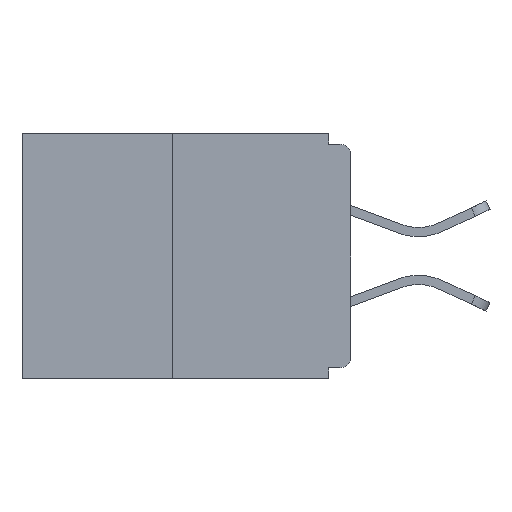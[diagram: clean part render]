
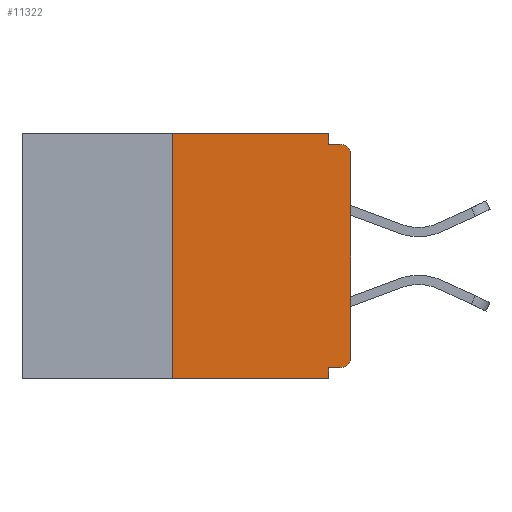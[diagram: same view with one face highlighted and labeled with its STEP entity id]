
A CAD part, left-side view. The second image highlights one B-rep face of the part: STEP entity #11322.
In plain terms, the highlighted planar face has unit normal (-1, 0, 0).
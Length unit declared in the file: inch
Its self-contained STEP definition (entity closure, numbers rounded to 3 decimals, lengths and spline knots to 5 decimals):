
#117 = DIRECTION ( 'NONE',  ( -1., 0., 0. ) ) ;
#404 = AXIS2_PLACEMENT_3D ( 'NONE', #14959, #117, #7440 ) ;
#451 = ORIENTED_EDGE ( 'NONE', *, *, #8232, .F. ) ;
#1149 = ORIENTED_EDGE ( 'NONE', *, *, #3819, .F. ) ;
#1339 = ORIENTED_EDGE ( 'NONE', *, *, #10463, .T. ) ;
#1766 = VERTEX_POINT ( 'NONE', #9526 ) ;
#1997 = VERTEX_POINT ( 'NONE', #14648 ) ;
#2332 = EDGE_CURVE ( 'NONE', #9503, #16705, #18944, .T. ) ;
#2663 = EDGE_LOOP ( 'NONE', ( #12184, #16238, #3317, #6544, #1149, #1339, #11304, #2722, #451, #3646 ) ) ;
#2677 = CARTESIAN_POINT ( 'NONE',  ( 0., 0.031, -0.328 ) ) ;
#2722 = ORIENTED_EDGE ( 'NONE', *, *, #17305, .T. ) ;
#2794 = CARTESIAN_POINT ( 'NONE',  ( 0., 0.46, -0.343 ) ) ;
#2967 = VERTEX_POINT ( 'NONE', #2677 ) ;
#3242 = VECTOR ( 'NONE', #5401, 39.37008 ) ;
#3317 = ORIENTED_EDGE ( 'NONE', *, *, #12271, .T. ) ;
#3443 = AXIS2_PLACEMENT_3D ( 'NONE', #6434, #9152, #13773 ) ;
#3646 = ORIENTED_EDGE ( 'NONE', *, *, #4870, .F. ) ;
#3714 = VERTEX_POINT ( 'NONE', #4981 ) ;
#3819 = EDGE_CURVE ( 'NONE', #1997, #2967, #16597, .T. ) ;
#4604 = CARTESIAN_POINT ( 'NONE',  ( 0., 0.031, -0.015 ) ) ;
#4810 = DIRECTION ( 'NONE',  ( 0., -1., 0. ) ) ;
#4870 = EDGE_CURVE ( 'NONE', #1766, #17278, #15366, .T. ) ;
#4981 = CARTESIAN_POINT ( 'NONE',  ( 0., 0., -0.313 ) ) ;
#5036 = CARTESIAN_POINT ( 'NONE',  ( 0., 0.031, -0.343 ) ) ;
#5191 = DIRECTION ( 'NONE',  ( 0., 0., 1. ) ) ;
#5307 = VERTEX_POINT ( 'NONE', #18093 ) ;
#5401 = DIRECTION ( 'NONE',  ( 0., -1., 0. ) ) ;
#5493 = VECTOR ( 'NONE', #6593, 39.37008 ) ;
#5878 = CARTESIAN_POINT ( 'NONE',  ( 0., 0.25, 0. ) ) ;
#6434 = CARTESIAN_POINT ( 'NONE',  ( 0., 0.015, -0.03 ) ) ;
#6523 = CARTESIAN_POINT ( 'NONE',  ( 0., 0.031, 0. ) ) ;
#6544 = ORIENTED_EDGE ( 'NONE', *, *, #14697, .F. ) ;
#6593 = DIRECTION ( 'NONE',  ( 0., 0., -1. ) ) ;
#7440 = DIRECTION ( 'NONE',  ( 0., 0., -1. ) ) ;
#7446 = AXIS2_PLACEMENT_3D ( 'NONE', #12922, #14546, #10168 ) ;
#7646 = LINE ( 'NONE', #14327, #3242 ) ;
#7720 = CARTESIAN_POINT ( 'NONE',  ( 0., 0., -0.015 ) ) ;
#8051 = CIRCLE ( 'NONE', #3443, 0.015 ) ;
#8120 = VECTOR ( 'NONE', #15920, 39.37008 ) ;
#8232 = EDGE_CURVE ( 'NONE', #17278, #5307, #15681, .T. ) ;
#8973 = VECTOR ( 'NONE', #17802, 39.37008 ) ;
#9098 = EDGE_CURVE ( 'NONE', #16705, #1766, #7646, .T. ) ;
#9130 = LINE ( 'NONE', #18225, #18767 ) ;
#9152 = DIRECTION ( 'NONE',  ( -1., 0., 0. ) ) ;
#9433 = LINE ( 'NONE', #14816, #8973 ) ;
#9503 = VERTEX_POINT ( 'NONE', #17490 ) ;
#9526 = CARTESIAN_POINT ( 'NONE',  ( 0., 0.031, 0. ) ) ;
#10168 = DIRECTION ( 'NONE',  ( 0., 0., -1. ) ) ;
#10463 = EDGE_CURVE ( 'NONE', #1997, #3714, #18842, .T. ) ;
#10589 = VERTEX_POINT ( 'NONE', #5036 ) ;
#10707 = FACE_OUTER_BOUND ( 'NONE', #2663, .T. ) ;
#11304 = ORIENTED_EDGE ( 'NONE', *, *, #18548, .T. ) ;
#11322 = ADVANCED_FACE ( 'NONE', ( #10707 ), #17408, .F. ) ;
#11354 = VECTOR ( 'NONE', #11773, 39.37008 ) ;
#11773 = DIRECTION ( 'NONE',  ( 0., 0., 1. ) ) ;
#12184 = ORIENTED_EDGE ( 'NONE', *, *, #9098, .F. ) ;
#12271 = EDGE_CURVE ( 'NONE', #9503, #10589, #17094, .T. ) ;
#12639 = CARTESIAN_POINT ( 'NONE',  ( 0., 0., -0.03 ) ) ;
#12886 = CARTESIAN_POINT ( 'NONE',  ( 0., 0.25, 0. ) ) ;
#12922 = CARTESIAN_POINT ( 'NONE',  ( 0., 0.46, 0. ) ) ;
#13773 = DIRECTION ( 'NONE',  ( 0., 0., -1. ) ) ;
#14327 = CARTESIAN_POINT ( 'NONE',  ( 0., 0.46, 0. ) ) ;
#14546 = DIRECTION ( 'NONE',  ( 1., 0., 0. ) ) ;
#14590 = CARTESIAN_POINT ( 'NONE',  ( 0., 0., -0.328 ) ) ;
#14591 = VECTOR ( 'NONE', #15901, 39.37008 ) ;
#14648 = CARTESIAN_POINT ( 'NONE',  ( 0., 0.015, -0.328 ) ) ;
#14697 = EDGE_CURVE ( 'NONE', #2967, #10589, #9433, .T. ) ;
#14816 = CARTESIAN_POINT ( 'NONE',  ( 0., 0.031, -0.343 ) ) ;
#14959 = CARTESIAN_POINT ( 'NONE',  ( 0., 0.015, -0.313 ) ) ;
#15366 = LINE ( 'NONE', #6523, #5493 ) ;
#15681 = LINE ( 'NONE', #7720, #16832 ) ;
#15901 = DIRECTION ( 'NONE',  ( 0., -1., 0. ) ) ;
#15920 = DIRECTION ( 'NONE',  ( 0., 1., 0. ) ) ;
#16238 = ORIENTED_EDGE ( 'NONE', *, *, #2332, .F. ) ;
#16597 = LINE ( 'NONE', #14590, #8120 ) ;
#16705 = VERTEX_POINT ( 'NONE', #12886 ) ;
#16832 = VECTOR ( 'NONE', #4810, 39.37008 ) ;
#17094 = LINE ( 'NONE', #2794, #14591 ) ;
#17278 = VERTEX_POINT ( 'NONE', #4604 ) ;
#17305 = EDGE_CURVE ( 'NONE', #18595, #5307, #8051, .T. ) ;
#17408 = PLANE ( 'NONE',  #7446 ) ;
#17490 = CARTESIAN_POINT ( 'NONE',  ( 0., 0.25, -0.343 ) ) ;
#17802 = DIRECTION ( 'NONE',  ( 0., 0., -1. ) ) ;
#18093 = CARTESIAN_POINT ( 'NONE',  ( 0., 0.015, -0.015 ) ) ;
#18225 = CARTESIAN_POINT ( 'NONE',  ( 0., 0., 0. ) ) ;
#18548 = EDGE_CURVE ( 'NONE', #3714, #18595, #9130, .T. ) ;
#18595 = VERTEX_POINT ( 'NONE', #12639 ) ;
#18767 = VECTOR ( 'NONE', #5191, 39.37008 ) ;
#18842 = CIRCLE ( 'NONE', #404, 0.015 ) ;
#18944 = LINE ( 'NONE', #5878, #11354 ) ;
